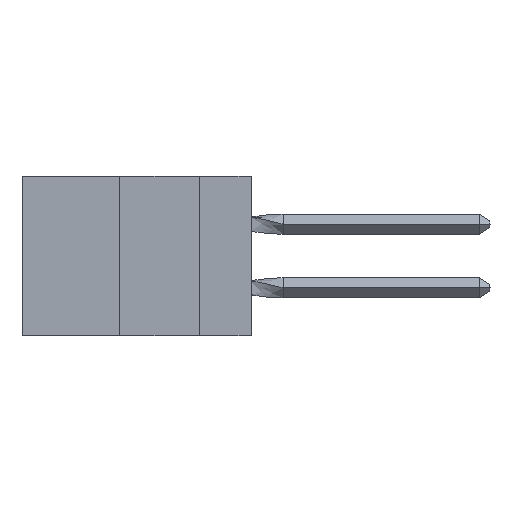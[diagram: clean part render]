
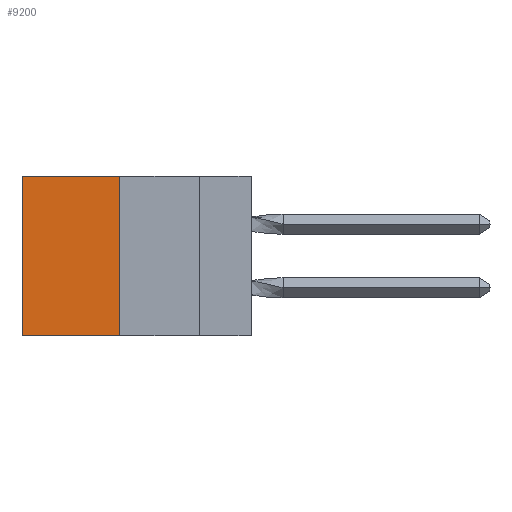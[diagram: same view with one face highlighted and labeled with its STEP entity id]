
A CAD part, left-side view. The second image highlights one B-rep face of the part: STEP entity #9200.
In plain terms, the highlighted planar face has unit normal (-1, 0, 0).
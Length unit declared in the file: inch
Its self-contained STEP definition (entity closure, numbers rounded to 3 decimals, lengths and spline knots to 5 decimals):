
#72 = DIRECTION ( 'NONE',  ( 0., 1., 0. ) ) ;
#85 = DIRECTION ( 'NONE',  ( 0., 1., 0. ) ) ;
#303 = ORIENTED_EDGE ( 'NONE', *, *, #7162, .F. ) ;
#1597 = LINE ( 'NONE', #3413, #10117 ) ;
#1719 = VERTEX_POINT ( 'NONE', #2900 ) ;
#2303 = CARTESIAN_POINT ( 'NONE',  ( 0.305, 0.72, 0. ) ) ;
#2646 = FACE_OUTER_BOUND ( 'NONE', #8692, .T. ) ;
#2900 = CARTESIAN_POINT ( 'NONE',  ( 0.305, 0.413, -0.5 ) ) ;
#3413 = CARTESIAN_POINT ( 'NONE',  ( 0.305, 0.413, -0.5 ) ) ;
#3529 = CARTESIAN_POINT ( 'NONE',  ( 0.305, 0.413, 0. ) ) ;
#3540 = EDGE_CURVE ( 'NONE', #1719, #10164, #6161, .T. ) ;
#4432 = EDGE_CURVE ( 'NONE', #7742, #10164, #9813, .T. ) ;
#5283 = DIRECTION ( 'NONE',  ( 1., 0., 0. ) ) ;
#5981 = CARTESIAN_POINT ( 'NONE',  ( 0.305, 0.413, -0.5 ) ) ;
#6161 = LINE ( 'NONE', #5981, #11863 ) ;
#6164 = VECTOR ( 'NONE', #72, 39.37008 ) ;
#6435 = DIRECTION ( 'NONE',  ( 0., 0., -1. ) ) ;
#6653 = AXIS2_PLACEMENT_3D ( 'NONE', #9941, #5283, #6435 ) ;
#7162 = EDGE_CURVE ( 'NONE', #10755, #1719, #1597, .T. ) ;
#7742 = VERTEX_POINT ( 'NONE', #2303 ) ;
#7777 = PLANE ( 'NONE',  #6653 ) ;
#8028 = ORIENTED_EDGE ( 'NONE', *, *, #3540, .F. ) ;
#8692 = EDGE_LOOP ( 'NONE', ( #11037, #8028, #303, #11228 ) ) ;
#9075 = DIRECTION ( 'NONE',  ( 0., 0., -1. ) ) ;
#9200 = ADVANCED_FACE ( 'NONE', ( #2646 ), #7777, .F. ) ;
#9228 = CARTESIAN_POINT ( 'NONE',  ( 0.305, 0.72, -0.5 ) ) ;
#9813 = LINE ( 'NONE', #11287, #13503 ) ;
#9941 = CARTESIAN_POINT ( 'NONE',  ( 0.305, 0.413, -0.5 ) ) ;
#10117 = VECTOR ( 'NONE', #11736, 39.37008 ) ;
#10164 = VERTEX_POINT ( 'NONE', #9228 ) ;
#10751 = LINE ( 'NONE', #3529, #6164 ) ;
#10755 = VERTEX_POINT ( 'NONE', #12960 ) ;
#11037 = ORIENTED_EDGE ( 'NONE', *, *, #4432, .T. ) ;
#11228 = ORIENTED_EDGE ( 'NONE', *, *, #14924, .T. ) ;
#11287 = CARTESIAN_POINT ( 'NONE',  ( 0.305, 0.72, -0.5 ) ) ;
#11736 = DIRECTION ( 'NONE',  ( 0., 0., -1. ) ) ;
#11863 = VECTOR ( 'NONE', #85, 39.37008 ) ;
#12960 = CARTESIAN_POINT ( 'NONE',  ( 0.305, 0.413, 0. ) ) ;
#13503 = VECTOR ( 'NONE', #9075, 39.37008 ) ;
#14924 = EDGE_CURVE ( 'NONE', #10755, #7742, #10751, .T. ) ;
